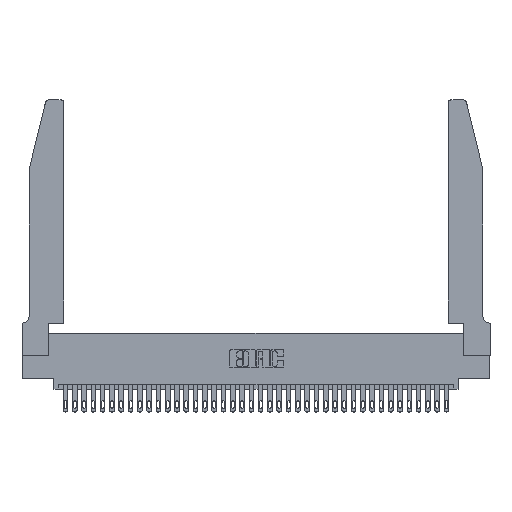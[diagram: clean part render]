
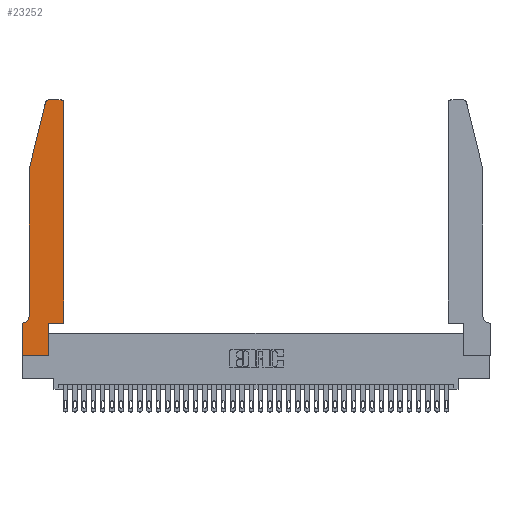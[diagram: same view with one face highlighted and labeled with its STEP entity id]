
A CAD part, top view. The second image highlights one B-rep face of the part: STEP entity #23252.
In plain terms, the highlighted planar face has unit normal (0, 0, 1).
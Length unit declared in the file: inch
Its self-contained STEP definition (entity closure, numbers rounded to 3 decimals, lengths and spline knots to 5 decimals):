
#274 = CARTESIAN_POINT ( 'NONE',  ( 0.0755, 2., 0.37 ) ) ;
#536 = CARTESIAN_POINT ( 'NONE',  ( 0.0055, 0.35, 0.37 ) ) ;
#579 = EDGE_CURVE ( 'NONE', #8677, #27126, #21731, .T. ) ;
#678 = VECTOR ( 'NONE', #36190, 39.37008 ) ;
#745 = DIRECTION ( 'NONE',  ( 0., 0., -1. ) ) ;
#1687 = CARTESIAN_POINT ( 'NONE',  ( 0., 0., 0.37 ) ) ;
#1786 = VERTEX_POINT ( 'NONE', #274 ) ;
#1963 = EDGE_CURVE ( 'NONE', #27126, #1786, #23058, .T. ) ;
#2011 = FACE_OUTER_BOUND ( 'NONE', #34667, .T. ) ;
#2428 = VECTOR ( 'NONE', #4677, 39.37008 ) ;
#2698 = VECTOR ( 'NONE', #23723, 39.37008 ) ;
#2943 = CARTESIAN_POINT ( 'NONE',  ( 0.4205, 2.72, 0.37 ) ) ;
#3222 = CARTESIAN_POINT ( 'NONE',  ( 0.0755, 2., 0.37 ) ) ;
#3290 = ORIENTED_EDGE ( 'NONE', *, *, #21446, .T. ) ;
#4116 = CARTESIAN_POINT ( 'NONE',  ( 0.0755, 0.42, 0.37 ) ) ;
#4244 = AXIS2_PLACEMENT_3D ( 'NONE', #18260, #745, #21186 ) ;
#4677 = DIRECTION ( 'NONE',  ( 0., 1., 0. ) ) ;
#4687 = VERTEX_POINT ( 'NONE', #24506 ) ;
#4693 = VECTOR ( 'NONE', #11416, 39.37008 ) ;
#5112 = PLANE ( 'NONE',  #9049 ) ;
#7044 = DIRECTION ( 'NONE',  ( 1., 0., 0. ) ) ;
#7775 = CIRCLE ( 'NONE', #22163, 0.03 ) ;
#7899 = ORIENTED_EDGE ( 'NONE', *, *, #26372, .T. ) ;
#8032 = CARTESIAN_POINT ( 'NONE',  ( 0., 0.35, 0.37 ) ) ;
#8491 = LINE ( 'NONE', #36457, #678 ) ;
#8556 = DIRECTION ( 'NONE',  ( 1., 0., 0. ) ) ;
#8677 = VERTEX_POINT ( 'NONE', #33271 ) ;
#9049 = AXIS2_PLACEMENT_3D ( 'NONE', #8032, #22956, #19525 ) ;
#9540 = DIRECTION ( 'NONE',  ( 0., 0., 1. ) ) ;
#9664 = ORIENTED_EDGE ( 'NONE', *, *, #12753, .T. ) ;
#10417 = ORIENTED_EDGE ( 'NONE', *, *, #579, .T. ) ;
#10647 = CARTESIAN_POINT ( 'NONE',  ( 0.4505, 0.35, 0.37 ) ) ;
#11416 = DIRECTION ( 'NONE',  ( 1., 0., 0. ) ) ;
#12439 = LINE ( 'NONE', #26450, #4693 ) ;
#12603 = AXIS2_PLACEMENT_3D ( 'NONE', #15269, #9540, #18343 ) ;
#12753 = EDGE_CURVE ( 'NONE', #32485, #30808, #12439, .T. ) ;
#12913 = VECTOR ( 'NONE', #26189, 39.37008 ) ;
#14356 = VECTOR ( 'NONE', #19502, 39.37008 ) ;
#14488 = VERTEX_POINT ( 'NONE', #21359 ) ;
#15269 = CARTESIAN_POINT ( 'NONE',  ( 0.284, 2.72, 0.37 ) ) ;
#15433 = EDGE_CURVE ( 'NONE', #31382, #27086, #24115, .T. ) ;
#15562 = VECTOR ( 'NONE', #33960, 39.37008 ) ;
#15850 = CARTESIAN_POINT ( 'NONE',  ( 0.25487, 2.72718, 0.37 ) ) ;
#16355 = ORIENTED_EDGE ( 'NONE', *, *, #24574, .T. ) ;
#16561 = LINE ( 'NONE', #25343, #2428 ) ;
#16752 = LINE ( 'NONE', #1687, #21345 ) ;
#16920 = VERTEX_POINT ( 'NONE', #36180 ) ;
#17187 = VERTEX_POINT ( 'NONE', #22955 ) ;
#18260 = CARTESIAN_POINT ( 'NONE',  ( 0.0055, 0.42, 0.37 ) ) ;
#18343 = DIRECTION ( 'NONE',  ( 1., 0., 0. ) ) ;
#18356 = EDGE_CURVE ( 'NONE', #16920, #8677, #23389, .T. ) ;
#19502 = DIRECTION ( 'NONE',  ( -0.239, -0.971, 0. ) ) ;
#19525 = DIRECTION ( 'NONE',  ( 1., 0., 0. ) ) ;
#19552 = DIRECTION ( 'NONE',  ( 0., 1., 0. ) ) ;
#20046 = EDGE_CURVE ( 'NONE', #17187, #16920, #7775, .T. ) ;
#20260 = CARTESIAN_POINT ( 'NONE',  ( 0.0755, 0.35, 0.37 ) ) ;
#21186 = DIRECTION ( 'NONE',  ( -1., 0., 0. ) ) ;
#21345 = VECTOR ( 'NONE', #7044, 39.37008 ) ;
#21359 = CARTESIAN_POINT ( 'NONE',  ( 0., 0., 0.37 ) ) ;
#21446 = EDGE_CURVE ( 'NONE', #14488, #26671, #16752, .T. ) ;
#21534 = EDGE_CURVE ( 'NONE', #26671, #32485, #35910, .T. ) ;
#21731 = CIRCLE ( 'NONE', #12603, 0.03 ) ;
#22163 = AXIS2_PLACEMENT_3D ( 'NONE', #2943, #37596, #8556 ) ;
#22955 = CARTESIAN_POINT ( 'NONE',  ( 0.4505, 2.72, 0.37 ) ) ;
#22956 = DIRECTION ( 'NONE',  ( 0., 0., 1. ) ) ;
#23058 = LINE ( 'NONE', #28035, #14356 ) ;
#23252 = ADVANCED_FACE ( 'NONE', ( #2011 ), #5112, .T. ) ;
#23389 = LINE ( 'NONE', #24918, #15562 ) ;
#23723 = DIRECTION ( 'NONE',  ( -1., 0., 0. ) ) ;
#23795 = EDGE_CURVE ( 'NONE', #30808, #17187, #16561, .T. ) ;
#23862 = CARTESIAN_POINT ( 'NONE',  ( 0.2865, 0., 0.37 ) ) ;
#24115 = CIRCLE ( 'NONE', #4244, 0.07 ) ;
#24337 = ORIENTED_EDGE ( 'NONE', *, *, #30291, .T. ) ;
#24506 = CARTESIAN_POINT ( 'NONE',  ( 0., 0.35, 0.37 ) ) ;
#24574 = EDGE_CURVE ( 'NONE', #1786, #31382, #32599, .T. ) ;
#24918 = CARTESIAN_POINT ( 'NONE',  ( 0.2605, 2.75, 0.37 ) ) ;
#25343 = CARTESIAN_POINT ( 'NONE',  ( 0.4505, 0.35, 0.37 ) ) ;
#26189 = DIRECTION ( 'NONE',  ( 0., -1., 0. ) ) ;
#26372 = EDGE_CURVE ( 'NONE', #4687, #14488, #8491, .T. ) ;
#26450 = CARTESIAN_POINT ( 'NONE',  ( 0.4505, 0.35, 0.37 ) ) ;
#26671 = VERTEX_POINT ( 'NONE', #23862 ) ;
#27086 = VERTEX_POINT ( 'NONE', #536 ) ;
#27126 = VERTEX_POINT ( 'NONE', #15850 ) ;
#28035 = CARTESIAN_POINT ( 'NONE',  ( 0.0755, 2., 0.37 ) ) ;
#28199 = VECTOR ( 'NONE', #19552, 39.37008 ) ;
#28223 = CARTESIAN_POINT ( 'NONE',  ( 0.2865, 0.35, 0.37 ) ) ;
#30291 = EDGE_CURVE ( 'NONE', #27086, #4687, #32384, .T. ) ;
#30750 = ORIENTED_EDGE ( 'NONE', *, *, #15433, .T. ) ;
#30808 = VERTEX_POINT ( 'NONE', #10647 ) ;
#31382 = VERTEX_POINT ( 'NONE', #4116 ) ;
#31442 = ORIENTED_EDGE ( 'NONE', *, *, #20046, .T. ) ;
#31458 = ORIENTED_EDGE ( 'NONE', *, *, #21534, .T. ) ;
#32384 = LINE ( 'NONE', #20260, #2698 ) ;
#32485 = VERTEX_POINT ( 'NONE', #37291 ) ;
#32599 = LINE ( 'NONE', #3222, #12913 ) ;
#33271 = CARTESIAN_POINT ( 'NONE',  ( 0.284, 2.75, 0.37 ) ) ;
#33960 = DIRECTION ( 'NONE',  ( -1., 0., 0. ) ) ;
#34657 = ORIENTED_EDGE ( 'NONE', *, *, #23795, .T. ) ;
#34667 = EDGE_LOOP ( 'NONE', ( #35534, #10417, #37299, #16355, #30750, #24337, #7899, #3290, #31458, #9664, #34657, #31442 ) ) ;
#35534 = ORIENTED_EDGE ( 'NONE', *, *, #18356, .T. ) ;
#35910 = LINE ( 'NONE', #28223, #28199 ) ;
#36180 = CARTESIAN_POINT ( 'NONE',  ( 0.4205, 2.75, 0.37 ) ) ;
#36190 = DIRECTION ( 'NONE',  ( 0., -1., 0. ) ) ;
#36457 = CARTESIAN_POINT ( 'NONE',  ( 0., 0., 0.37 ) ) ;
#37291 = CARTESIAN_POINT ( 'NONE',  ( 0.2865, 0.35, 0.37 ) ) ;
#37299 = ORIENTED_EDGE ( 'NONE', *, *, #1963, .T. ) ;
#37596 = DIRECTION ( 'NONE',  ( 0., 0., 1. ) ) ;
